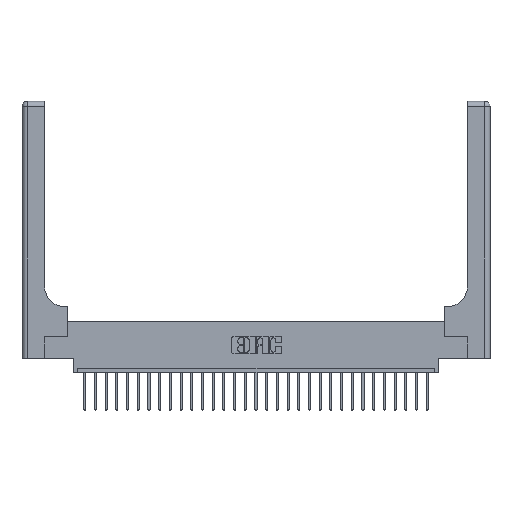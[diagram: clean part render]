
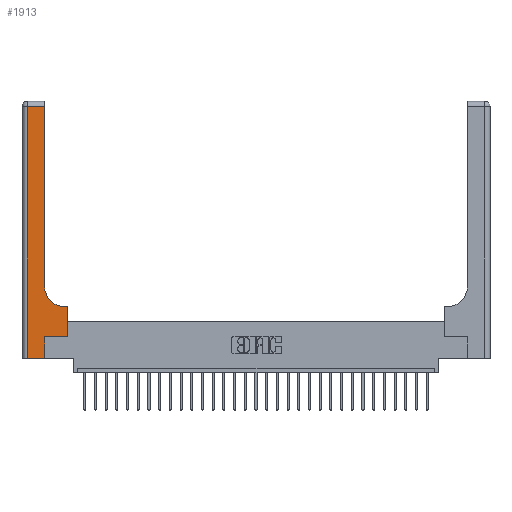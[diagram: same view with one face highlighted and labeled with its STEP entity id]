
A CAD part, top view. The second image highlights one B-rep face of the part: STEP entity #1913.
In plain terms, the highlighted planar face has unit normal (0, 0, 1).
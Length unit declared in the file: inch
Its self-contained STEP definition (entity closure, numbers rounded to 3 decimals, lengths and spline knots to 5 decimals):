
#132 = CARTESIAN_POINT ( 'NONE',  ( 0.51, 0.85, 0.37 ) ) ;
#430 = DIRECTION ( 'NONE',  ( 1., 0., 0. ) ) ;
#693 = ORIENTED_EDGE ( 'NONE', *, *, #17549, .T. ) ;
#784 = CARTESIAN_POINT ( 'NONE',  ( 0.528, 0.6, 0.37 ) ) ;
#1302 = EDGE_LOOP ( 'NONE', ( #18970, #15644, #10760, #20217, #20322, #19324, #17317, #19768, #693 ) ) ;
#1504 = DIRECTION ( 'NONE',  ( 0., -1., 0. ) ) ;
#1523 = VECTOR ( 'NONE', #11320, 39.37008 ) ;
#1584 = VECTOR ( 'NONE', #6083, 39.37008 ) ;
#1650 = CARTESIAN_POINT ( 'NONE',  ( 0., 0., 0.37 ) ) ;
#1736 = LINE ( 'NONE', #5971, #26548 ) ;
#1822 = LINE ( 'NONE', #3847, #8975 ) ;
#1913 = ADVANCED_FACE ( 'NONE', ( #23763 ), #2721, .F. ) ;
#2567 = VERTEX_POINT ( 'NONE', #24911 ) ;
#2721 = PLANE ( 'NONE',  #9568 ) ;
#3137 = CARTESIAN_POINT ( 'NONE',  ( 0.51, 0.6, 0.37 ) ) ;
#3466 = CARTESIAN_POINT ( 'NONE',  ( 0.528, 0.25, 0.37 ) ) ;
#3648 = DIRECTION ( 'NONE',  ( -1., 0., 0. ) ) ;
#3847 = CARTESIAN_POINT ( 'NONE',  ( 0.06, 3., 0.37 ) ) ;
#4345 = DIRECTION ( 'NONE',  ( 0., 0., -1. ) ) ;
#5127 = LINE ( 'NONE', #25439, #11003 ) ;
#5283 = EDGE_CURVE ( 'NONE', #11665, #7362, #5470, .T. ) ;
#5470 = LINE ( 'NONE', #7289, #24770 ) ;
#5971 = CARTESIAN_POINT ( 'NONE',  ( 0.528, 0.25, 0.37 ) ) ;
#6083 = DIRECTION ( 'NONE',  ( 1., 0., 0. ) ) ;
#6739 = VERTEX_POINT ( 'NONE', #20085 ) ;
#6784 = LINE ( 'NONE', #1650, #1584 ) ;
#7070 = LINE ( 'NONE', #23847, #1523 ) ;
#7289 = CARTESIAN_POINT ( 'NONE',  ( 0.26, 3., 0.37 ) ) ;
#7362 = VERTEX_POINT ( 'NONE', #9188 ) ;
#8509 = VERTEX_POINT ( 'NONE', #23839 ) ;
#8975 = VECTOR ( 'NONE', #1504, 39.37008 ) ;
#9188 = CARTESIAN_POINT ( 'NONE',  ( 0.26, 2.94, 0.37 ) ) ;
#9568 = AXIS2_PLACEMENT_3D ( 'NONE', #13085, #4345, #18944 ) ;
#10344 = DIRECTION ( 'NONE',  ( 0., 1., 0. ) ) ;
#10760 = ORIENTED_EDGE ( 'NONE', *, *, #13937, .T. ) ;
#11003 = VECTOR ( 'NONE', #430, 39.37008 ) ;
#11188 = VERTEX_POINT ( 'NONE', #784 ) ;
#11320 = DIRECTION ( 'NONE',  ( 0., 1., 0. ) ) ;
#11398 = EDGE_CURVE ( 'NONE', #11188, #26829, #17589, .T. ) ;
#11665 = VERTEX_POINT ( 'NONE', #26029 ) ;
#12024 = EDGE_CURVE ( 'NONE', #21338, #6739, #6784, .T. ) ;
#12637 = CARTESIAN_POINT ( 'NONE',  ( 0., 2.94, 0.37 ) ) ;
#12964 = EDGE_CURVE ( 'NONE', #7362, #2567, #18475, .T. ) ;
#13085 = CARTESIAN_POINT ( 'NONE',  ( 0., 3., 0.37 ) ) ;
#13937 = EDGE_CURVE ( 'NONE', #2567, #21338, #1822, .T. ) ;
#14300 = VECTOR ( 'NONE', #3648, 39.37008 ) ;
#14309 = AXIS2_PLACEMENT_3D ( 'NONE', #132, #14399, #22749 ) ;
#14399 = DIRECTION ( 'NONE',  ( 0., 0., -1. ) ) ;
#14817 = DIRECTION ( 'NONE',  ( -1., 0., 0. ) ) ;
#15644 = ORIENTED_EDGE ( 'NONE', *, *, #12964, .T. ) ;
#16141 = CARTESIAN_POINT ( 'NONE',  ( 0.26, 0.6, 0.37 ) ) ;
#16929 = EDGE_CURVE ( 'NONE', #26090, #11188, #1736, .T. ) ;
#17317 = ORIENTED_EDGE ( 'NONE', *, *, #16929, .T. ) ;
#17549 = EDGE_CURVE ( 'NONE', #26829, #11665, #24227, .T. ) ;
#17589 = LINE ( 'NONE', #16141, #14300 ) ;
#17946 = DIRECTION ( 'NONE',  ( 0., 1., 0. ) ) ;
#18153 = VECTOR ( 'NONE', #14817, 39.37008 ) ;
#18475 = LINE ( 'NONE', #12637, #18153 ) ;
#18944 = DIRECTION ( 'NONE',  ( -1., 0., 0. ) ) ;
#18970 = ORIENTED_EDGE ( 'NONE', *, *, #5283, .T. ) ;
#19324 = ORIENTED_EDGE ( 'NONE', *, *, #19951, .T. ) ;
#19768 = ORIENTED_EDGE ( 'NONE', *, *, #11398, .T. ) ;
#19951 = EDGE_CURVE ( 'NONE', #8509, #26090, #5127, .T. ) ;
#20085 = CARTESIAN_POINT ( 'NONE',  ( 0.265, 0., 0.37 ) ) ;
#20217 = ORIENTED_EDGE ( 'NONE', *, *, #12024, .T. ) ;
#20322 = ORIENTED_EDGE ( 'NONE', *, *, #21097, .T. ) ;
#21097 = EDGE_CURVE ( 'NONE', #6739, #8509, #7070, .T. ) ;
#21338 = VERTEX_POINT ( 'NONE', #24836 ) ;
#22749 = DIRECTION ( 'NONE',  ( 1., 0., 0. ) ) ;
#23763 = FACE_OUTER_BOUND ( 'NONE', #1302, .T. ) ;
#23839 = CARTESIAN_POINT ( 'NONE',  ( 0.265, 0.25, 0.37 ) ) ;
#23847 = CARTESIAN_POINT ( 'NONE',  ( 0.265, 0., 0.37 ) ) ;
#24227 = CIRCLE ( 'NONE', #14309, 0.25 ) ;
#24770 = VECTOR ( 'NONE', #17946, 39.37008 ) ;
#24836 = CARTESIAN_POINT ( 'NONE',  ( 0.06, 0., 0.37 ) ) ;
#24911 = CARTESIAN_POINT ( 'NONE',  ( 0.06, 2.94, 0.37 ) ) ;
#25439 = CARTESIAN_POINT ( 'NONE',  ( 0.265, 0.25, 0.37 ) ) ;
#26029 = CARTESIAN_POINT ( 'NONE',  ( 0.26, 0.85, 0.37 ) ) ;
#26090 = VERTEX_POINT ( 'NONE', #3466 ) ;
#26548 = VECTOR ( 'NONE', #10344, 39.37008 ) ;
#26829 = VERTEX_POINT ( 'NONE', #3137 ) ;
